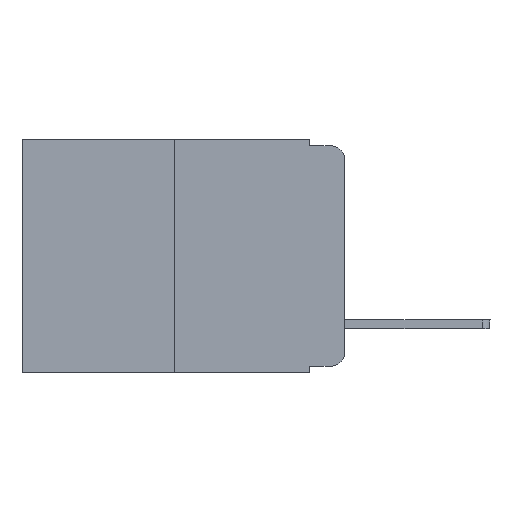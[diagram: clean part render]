
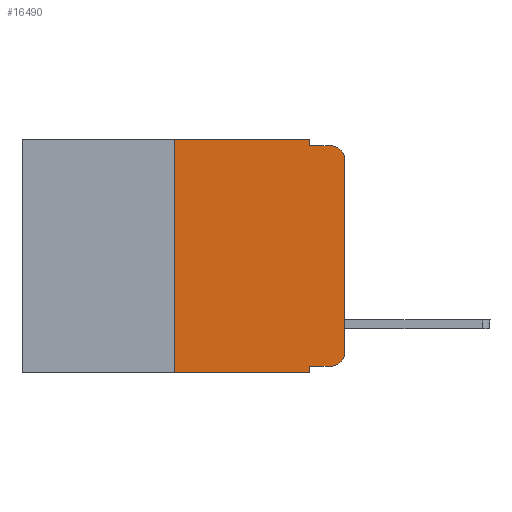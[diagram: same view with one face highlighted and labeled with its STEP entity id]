
A CAD part, left-side view. The second image highlights one B-rep face of the part: STEP entity #16490.
In plain terms, the highlighted planar face has unit normal (-1, 0, 0).
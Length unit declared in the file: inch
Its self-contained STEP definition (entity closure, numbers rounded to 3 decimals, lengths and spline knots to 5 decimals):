
#112 = CARTESIAN_POINT ( 'NONE',  ( 0., 0.25, -0.343 ) ) ;
#334 = LINE ( 'NONE', #16644, #1265 ) ;
#524 = DIRECTION ( 'NONE',  ( 0., 0., 1. ) ) ;
#907 = VECTOR ( 'NONE', #1080, 39.37008 ) ;
#1080 = DIRECTION ( 'NONE',  ( 0., 0., 1. ) ) ;
#1265 = VECTOR ( 'NONE', #16579, 39.37008 ) ;
#1458 = DIRECTION ( 'NONE',  ( 0., -1., 0. ) ) ;
#1665 = VECTOR ( 'NONE', #18917, 39.37008 ) ;
#1905 = EDGE_CURVE ( 'NONE', #3935, #3067, #334, .T. ) ;
#2395 = ORIENTED_EDGE ( 'NONE', *, *, #12269, .T. ) ;
#2711 = AXIS2_PLACEMENT_3D ( 'NONE', #11739, #4466, #4331 ) ;
#3067 = VERTEX_POINT ( 'NONE', #7660 ) ;
#3286 = LINE ( 'NONE', #18141, #14309 ) ;
#3300 = LINE ( 'NONE', #7070, #1665 ) ;
#3554 = ORIENTED_EDGE ( 'NONE', *, *, #8624, .T. ) ;
#3729 = VERTEX_POINT ( 'NONE', #6489 ) ;
#3935 = VERTEX_POINT ( 'NONE', #12982 ) ;
#4331 = DIRECTION ( 'NONE',  ( 0., 0., -1. ) ) ;
#4466 = DIRECTION ( 'NONE',  ( -1., 0., 0. ) ) ;
#4529 = DIRECTION ( 'NONE',  ( 0., 0., -1. ) ) ;
#4802 = LINE ( 'NONE', #13894, #16037 ) ;
#5385 = ORIENTED_EDGE ( 'NONE', *, *, #16366, .F. ) ;
#5397 = CARTESIAN_POINT ( 'NONE',  ( 0., 0.473, 0. ) ) ;
#5538 = ORIENTED_EDGE ( 'NONE', *, *, #8006, .F. ) ;
#6405 = ORIENTED_EDGE ( 'NONE', *, *, #7178, .T. ) ;
#6489 = CARTESIAN_POINT ( 'NONE',  ( 0., 0.051, -0.333 ) ) ;
#6495 = LINE ( 'NONE', #17250, #907 ) ;
#6610 = DIRECTION ( 'NONE',  ( 0., 0., -1. ) ) ;
#6636 = VECTOR ( 'NONE', #9435, 39.37008 ) ;
#6709 = VERTEX_POINT ( 'NONE', #10664 ) ;
#6747 = ORIENTED_EDGE ( 'NONE', *, *, #19080, .F. ) ;
#6804 = CARTESIAN_POINT ( 'NONE',  ( 0., 0.25, 0. ) ) ;
#6951 = ORIENTED_EDGE ( 'NONE', *, *, #1905, .F. ) ;
#7070 = CARTESIAN_POINT ( 'NONE',  ( 0., 0.051, 0. ) ) ;
#7178 = EDGE_CURVE ( 'NONE', #18005, #6709, #13345, .T. ) ;
#7432 = CARTESIAN_POINT ( 'NONE',  ( 0., 0.02, -0.333 ) ) ;
#7660 = CARTESIAN_POINT ( 'NONE',  ( 0., 0.02, -0.01 ) ) ;
#8006 = EDGE_CURVE ( 'NONE', #3729, #17007, #4802, .T. ) ;
#8026 = CARTESIAN_POINT ( 'NONE',  ( 0., 0.473, -0.343 ) ) ;
#8274 = LINE ( 'NONE', #17704, #11165 ) ;
#8479 = DIRECTION ( 'NONE',  ( 0., 0., -1. ) ) ;
#8624 = EDGE_CURVE ( 'NONE', #3729, #18005, #18343, .T. ) ;
#9191 = CARTESIAN_POINT ( 'NONE',  ( 0., 0.051, -0.333 ) ) ;
#9435 = DIRECTION ( 'NONE',  ( 0., -1., 0. ) ) ;
#9773 = EDGE_LOOP ( 'NONE', ( #2395, #17364, #6951, #5385, #6747, #16830, #15862, #5538, #3554, #6405 ) ) ;
#9939 = DIRECTION ( 'NONE',  ( 1., 0., 0. ) ) ;
#10474 = CIRCLE ( 'NONE', #17490, 0.02 ) ;
#10664 = CARTESIAN_POINT ( 'NONE',  ( 0., 0., -0.313 ) ) ;
#11165 = VECTOR ( 'NONE', #1458, 39.37008 ) ;
#11739 = CARTESIAN_POINT ( 'NONE',  ( 0., 0.02, -0.313 ) ) ;
#12269 = EDGE_CURVE ( 'NONE', #6709, #18108, #6495, .T. ) ;
#12308 = AXIS2_PLACEMENT_3D ( 'NONE', #5397, #9939, #8479 ) ;
#12581 = EDGE_CURVE ( 'NONE', #14785, #17007, #15147, .T. ) ;
#12982 = CARTESIAN_POINT ( 'NONE',  ( 0., 0.051, -0.01 ) ) ;
#13333 = DIRECTION ( 'NONE',  ( -1., 0., 0. ) ) ;
#13345 = CIRCLE ( 'NONE', #2711, 0.02 ) ;
#13546 = CARTESIAN_POINT ( 'NONE',  ( 0., 0., -0.03 ) ) ;
#13894 = CARTESIAN_POINT ( 'NONE',  ( 0., 0.051, 0. ) ) ;
#14124 = PLANE ( 'NONE',  #12308 ) ;
#14166 = CARTESIAN_POINT ( 'NONE',  ( 0., 0.051, -0.343 ) ) ;
#14309 = VECTOR ( 'NONE', #524, 39.37008 ) ;
#14785 = VERTEX_POINT ( 'NONE', #112 ) ;
#15147 = LINE ( 'NONE', #8026, #17204 ) ;
#15327 = DIRECTION ( 'NONE',  ( 0., -1., 0. ) ) ;
#15862 = ORIENTED_EDGE ( 'NONE', *, *, #12581, .T. ) ;
#16010 = CARTESIAN_POINT ( 'NONE',  ( 0., 0.02, -0.03 ) ) ;
#16037 = VECTOR ( 'NONE', #6610, 39.37008 ) ;
#16366 = EDGE_CURVE ( 'NONE', #17062, #3935, #3300, .T. ) ;
#16490 = ADVANCED_FACE ( 'NONE', ( #18720 ), #14124, .F. ) ;
#16579 = DIRECTION ( 'NONE',  ( 0., -1., 0. ) ) ;
#16644 = CARTESIAN_POINT ( 'NONE',  ( 0., 0.051, -0.01 ) ) ;
#16830 = ORIENTED_EDGE ( 'NONE', *, *, #17652, .F. ) ;
#17007 = VERTEX_POINT ( 'NONE', #14166 ) ;
#17048 = VERTEX_POINT ( 'NONE', #6804 ) ;
#17062 = VERTEX_POINT ( 'NONE', #18359 ) ;
#17204 = VECTOR ( 'NONE', #15327, 39.37008 ) ;
#17250 = CARTESIAN_POINT ( 'NONE',  ( 0., 0., 0. ) ) ;
#17340 = EDGE_CURVE ( 'NONE', #18108, #3067, #10474, .T. ) ;
#17364 = ORIENTED_EDGE ( 'NONE', *, *, #17340, .T. ) ;
#17490 = AXIS2_PLACEMENT_3D ( 'NONE', #16010, #13333, #4529 ) ;
#17652 = EDGE_CURVE ( 'NONE', #14785, #17048, #3286, .T. ) ;
#17704 = CARTESIAN_POINT ( 'NONE',  ( 0., 0.473, 0. ) ) ;
#18005 = VERTEX_POINT ( 'NONE', #7432 ) ;
#18108 = VERTEX_POINT ( 'NONE', #13546 ) ;
#18141 = CARTESIAN_POINT ( 'NONE',  ( 0., 0.25, 0. ) ) ;
#18343 = LINE ( 'NONE', #9191, #6636 ) ;
#18359 = CARTESIAN_POINT ( 'NONE',  ( 0., 0.051, 0. ) ) ;
#18720 = FACE_OUTER_BOUND ( 'NONE', #9773, .T. ) ;
#18917 = DIRECTION ( 'NONE',  ( 0., 0., -1. ) ) ;
#19080 = EDGE_CURVE ( 'NONE', #17048, #17062, #8274, .T. ) ;
